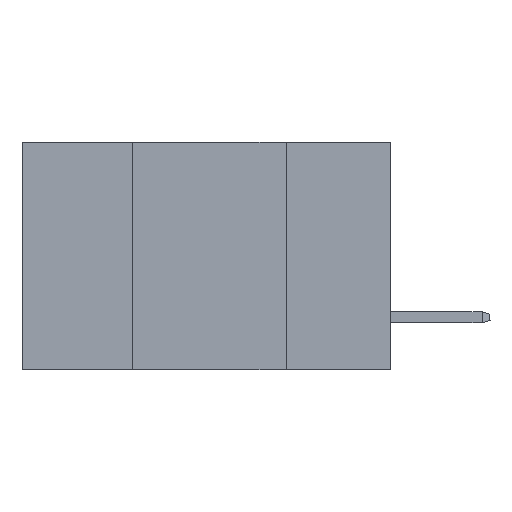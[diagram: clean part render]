
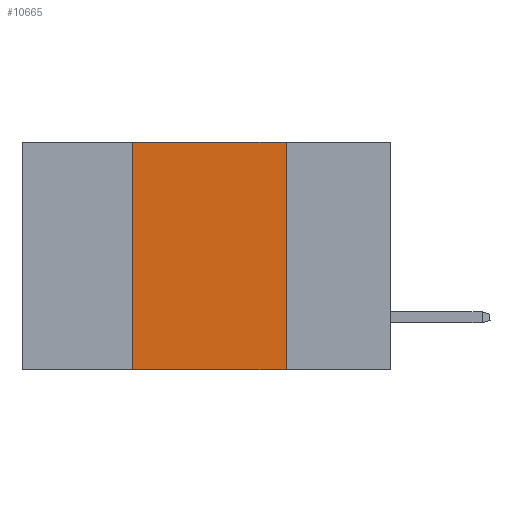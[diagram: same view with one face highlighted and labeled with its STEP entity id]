
A CAD part, left-side view. The second image highlights one B-rep face of the part: STEP entity #10665.
In plain terms, the highlighted planar face has unit normal (-1, 0, 0).
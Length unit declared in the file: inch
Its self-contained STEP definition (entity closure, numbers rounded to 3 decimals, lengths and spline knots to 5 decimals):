
#20 = VECTOR ( 'NONE', #11817, 39.37008 ) ;
#473 = CARTESIAN_POINT ( 'NONE',  ( 0., 0.42, 0. ) ) ;
#1012 = DIRECTION ( 'NONE',  ( 1., 0., 0. ) ) ;
#1243 = LINE ( 'NONE', #7246, #20 ) ;
#2072 = VECTOR ( 'NONE', #5113, 39.37008 ) ;
#2124 = DIRECTION ( 'NONE',  ( 0., 0., -1. ) ) ;
#3019 = ORIENTED_EDGE ( 'NONE', *, *, #11726, .F. ) ;
#3093 = EDGE_LOOP ( 'NONE', ( #13594, #3019, #12104, #3512 ) ) ;
#3110 = EDGE_CURVE ( 'NONE', #11619, #13771, #6864, .T. ) ;
#3355 = VERTEX_POINT ( 'NONE', #6261 ) ;
#3383 = EDGE_CURVE ( 'NONE', #3355, #13771, #1243, .T. ) ;
#3409 = CARTESIAN_POINT ( 'NONE',  ( 0., 0.42, 0. ) ) ;
#3512 = ORIENTED_EDGE ( 'NONE', *, *, #3110, .T. ) ;
#3712 = AXIS2_PLACEMENT_3D ( 'NONE', #7722, #1012, #2124 ) ;
#3862 = VECTOR ( 'NONE', #8734, 39.37008 ) ;
#4161 = CARTESIAN_POINT ( 'NONE',  ( 0., 0.6, -0.37 ) ) ;
#4341 = LINE ( 'NONE', #473, #2072 ) ;
#5113 = DIRECTION ( 'NONE',  ( 0., 0., 1. ) ) ;
#6261 = CARTESIAN_POINT ( 'NONE',  ( 0., 0.17, 0. ) ) ;
#6377 = CARTESIAN_POINT ( 'NONE',  ( 0., 0.6, 0. ) ) ;
#6514 = DIRECTION ( 'NONE',  ( 0., -1., 0. ) ) ;
#6864 = LINE ( 'NONE', #4161, #3862 ) ;
#7246 = CARTESIAN_POINT ( 'NONE',  ( 0., 0.17, 0. ) ) ;
#7722 = CARTESIAN_POINT ( 'NONE',  ( 0., 0.6, 0. ) ) ;
#8103 = VERTEX_POINT ( 'NONE', #3409 ) ;
#8734 = DIRECTION ( 'NONE',  ( 0., -1., 0. ) ) ;
#8874 = VECTOR ( 'NONE', #6514, 39.37008 ) ;
#9137 = EDGE_CURVE ( 'NONE', #11619, #8103, #4341, .T. ) ;
#10665 = ADVANCED_FACE ( 'NONE', ( #13472 ), #13301, .F. ) ;
#11619 = VERTEX_POINT ( 'NONE', #14125 ) ;
#11726 = EDGE_CURVE ( 'NONE', #8103, #3355, #12930, .T. ) ;
#11817 = DIRECTION ( 'NONE',  ( 0., 0., -1. ) ) ;
#12104 = ORIENTED_EDGE ( 'NONE', *, *, #9137, .F. ) ;
#12930 = LINE ( 'NONE', #6377, #8874 ) ;
#13301 = PLANE ( 'NONE',  #3712 ) ;
#13472 = FACE_OUTER_BOUND ( 'NONE', #3093, .T. ) ;
#13594 = ORIENTED_EDGE ( 'NONE', *, *, #3383, .F. ) ;
#13771 = VERTEX_POINT ( 'NONE', #14219 ) ;
#14125 = CARTESIAN_POINT ( 'NONE',  ( 0., 0.42, -0.37 ) ) ;
#14219 = CARTESIAN_POINT ( 'NONE',  ( 0., 0.17, -0.37 ) ) ;
